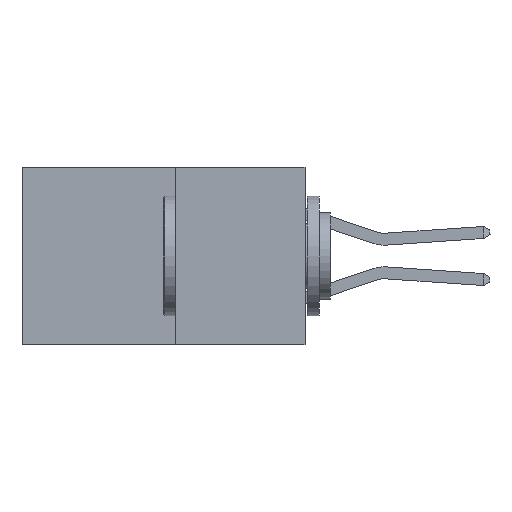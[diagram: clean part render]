
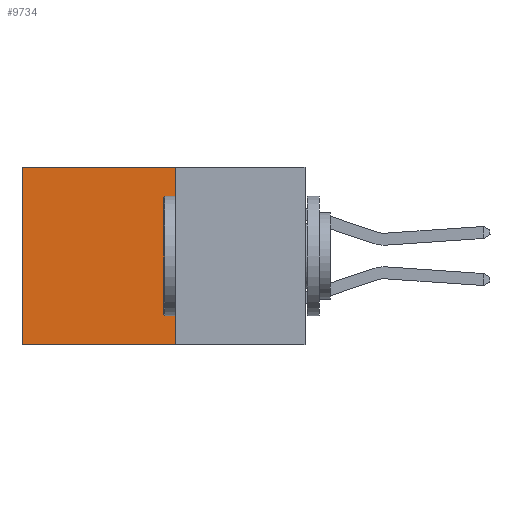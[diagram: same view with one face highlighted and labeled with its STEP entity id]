
A CAD part, left-side view. The second image highlights one B-rep face of the part: STEP entity #9734.
In plain terms, the highlighted planar face has unit normal (-1, 0, 0).
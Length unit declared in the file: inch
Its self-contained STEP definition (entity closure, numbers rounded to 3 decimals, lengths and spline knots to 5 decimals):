
#362 = EDGE_CURVE ( 'NONE', #909, #1790, #6525, .T. ) ;
#909 = VERTEX_POINT ( 'NONE', #5568 ) ;
#1669 = CARTESIAN_POINT ( 'NONE',  ( 0.277, 0.59, 0. ) ) ;
#1790 = VERTEX_POINT ( 'NONE', #3893 ) ;
#2483 = AXIS2_PLACEMENT_3D ( 'NONE', #4966, #11172, #5883 ) ;
#3648 = FACE_OUTER_BOUND ( 'NONE', #5345, .T. ) ;
#3672 = ORIENTED_EDGE ( 'NONE', *, *, #10805, .T. ) ;
#3765 = VECTOR ( 'NONE', #7450, 39.37008 ) ;
#3863 = CARTESIAN_POINT ( 'NONE',  ( 0.277, 0.59, -0.37 ) ) ;
#3893 = CARTESIAN_POINT ( 'NONE',  ( 0.277, 0.59, -0.37 ) ) ;
#4128 = VECTOR ( 'NONE', #9421, 39.37008 ) ;
#4315 = ORIENTED_EDGE ( 'NONE', *, *, #5001, .F. ) ;
#4601 = ORIENTED_EDGE ( 'NONE', *, *, #362, .F. ) ;
#4824 = DIRECTION ( 'NONE',  ( 0., 0., -1. ) ) ;
#4898 = CARTESIAN_POINT ( 'NONE',  ( 0.277, 0.27, -0.37 ) ) ;
#4966 = CARTESIAN_POINT ( 'NONE',  ( 0.277, 0.27, -0.37 ) ) ;
#5001 = EDGE_CURVE ( 'NONE', #8964, #909, #5720, .T. ) ;
#5097 = VECTOR ( 'NONE', #9625, 39.37008 ) ;
#5345 = EDGE_LOOP ( 'NONE', ( #3672, #4601, #4315, #11664 ) ) ;
#5568 = CARTESIAN_POINT ( 'NONE',  ( 0.277, 0.27, -0.37 ) ) ;
#5694 = CARTESIAN_POINT ( 'NONE',  ( 0.277, 0.27, 0. ) ) ;
#5720 = LINE ( 'NONE', #4898, #10187 ) ;
#5883 = DIRECTION ( 'NONE',  ( 0., 0., -1. ) ) ;
#6525 = LINE ( 'NONE', #10680, #4128 ) ;
#7450 = DIRECTION ( 'NONE',  ( 0., 0., -1. ) ) ;
#7470 = LINE ( 'NONE', #11301, #5097 ) ;
#7624 = PLANE ( 'NONE',  #2483 ) ;
#8964 = VERTEX_POINT ( 'NONE', #5694 ) ;
#9238 = EDGE_CURVE ( 'NONE', #8964, #11227, #7470, .T. ) ;
#9421 = DIRECTION ( 'NONE',  ( 0., 1., 0. ) ) ;
#9625 = DIRECTION ( 'NONE',  ( 0., 1., 0. ) ) ;
#9734 = ADVANCED_FACE ( 'NONE', ( #3648 ), #7624, .F. ) ;
#10187 = VECTOR ( 'NONE', #4824, 39.37008 ) ;
#10680 = CARTESIAN_POINT ( 'NONE',  ( 0.277, 0.27, -0.37 ) ) ;
#10805 = EDGE_CURVE ( 'NONE', #11227, #1790, #11161, .T. ) ;
#11161 = LINE ( 'NONE', #3863, #3765 ) ;
#11172 = DIRECTION ( 'NONE',  ( 1., 0., 0. ) ) ;
#11227 = VERTEX_POINT ( 'NONE', #1669 ) ;
#11301 = CARTESIAN_POINT ( 'NONE',  ( 0.277, 0.27, 0. ) ) ;
#11664 = ORIENTED_EDGE ( 'NONE', *, *, #9238, .T. ) ;
